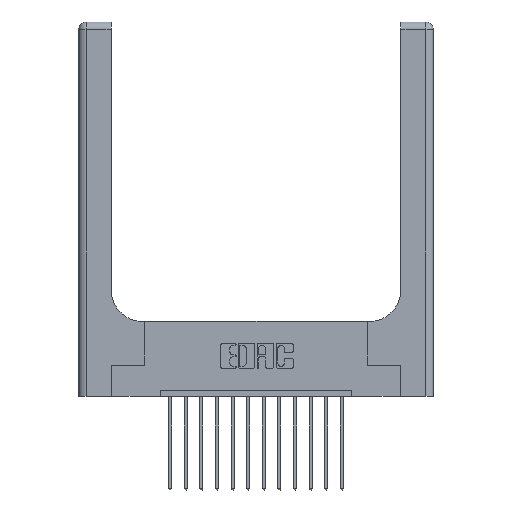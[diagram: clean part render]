
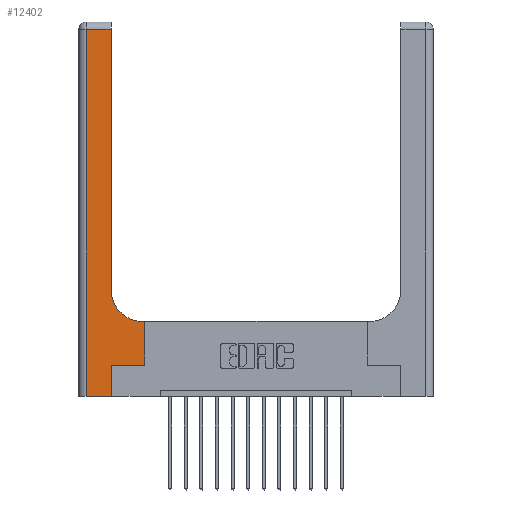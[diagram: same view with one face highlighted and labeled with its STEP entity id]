
A CAD part, top view. The second image highlights one B-rep face of the part: STEP entity #12402.
In plain terms, the highlighted planar face has unit normal (0, 0, 1).
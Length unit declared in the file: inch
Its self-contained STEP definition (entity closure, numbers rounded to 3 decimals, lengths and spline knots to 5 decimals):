
#96 = CARTESIAN_POINT ( 'NONE',  ( 0., 3., 0.37 ) ) ;
#171 = VERTEX_POINT ( 'NONE', #6019 ) ;
#181 = DIRECTION ( 'NONE',  ( 1., 0., 0. ) ) ;
#257 = EDGE_CURVE ( 'NONE', #2579, #5908, #6985, .T. ) ;
#1175 = LINE ( 'NONE', #15353, #2236 ) ;
#1240 = CARTESIAN_POINT ( 'NONE',  ( 0.528, 0.25, 0.37 ) ) ;
#1268 = CARTESIAN_POINT ( 'NONE',  ( 0.26, 2.94, 0.37 ) ) ;
#1392 = PLANE ( 'NONE',  #9883 ) ;
#1414 = ORIENTED_EDGE ( 'NONE', *, *, #13776, .T. ) ;
#1678 = LINE ( 'NONE', #4248, #4530 ) ;
#2134 = DIRECTION ( 'NONE',  ( 0., -1., 0. ) ) ;
#2166 = EDGE_CURVE ( 'NONE', #8527, #7662, #1175, .T. ) ;
#2236 = VECTOR ( 'NONE', #16609, 39.37008 ) ;
#2522 = VERTEX_POINT ( 'NONE', #14238 ) ;
#2579 = VERTEX_POINT ( 'NONE', #14970 ) ;
#2643 = CARTESIAN_POINT ( 'NONE',  ( 0.528, 0.25, 0.37 ) ) ;
#2962 = EDGE_CURVE ( 'NONE', #5908, #13254, #7901, .T. ) ;
#3064 = FACE_OUTER_BOUND ( 'NONE', #5101, .T. ) ;
#3127 = VECTOR ( 'NONE', #8066, 39.37008 ) ;
#3618 = VECTOR ( 'NONE', #3876, 39.37008 ) ;
#3773 = LINE ( 'NONE', #7328, #7438 ) ;
#3876 = DIRECTION ( 'NONE',  ( 0., 1., 0. ) ) ;
#4155 = EDGE_CURVE ( 'NONE', #171, #8527, #4359, .T. ) ;
#4224 = ORIENTED_EDGE ( 'NONE', *, *, #257, .T. ) ;
#4248 = CARTESIAN_POINT ( 'NONE',  ( 0., 0., 0.37 ) ) ;
#4333 = EDGE_CURVE ( 'NONE', #16553, #2522, #3773, .T. ) ;
#4359 = CIRCLE ( 'NONE', #16296, 0.25 ) ;
#4530 = VECTOR ( 'NONE', #14507, 39.37008 ) ;
#4594 = DIRECTION ( 'NONE',  ( 0., 1., 0. ) ) ;
#5101 = EDGE_LOOP ( 'NONE', ( #5566, #12782, #16397, #5996, #15455, #4224, #14226, #1414, #9257 ) ) ;
#5499 = DIRECTION ( 'NONE',  ( -1., 0., 0. ) ) ;
#5566 = ORIENTED_EDGE ( 'NONE', *, *, #2166, .T. ) ;
#5616 = CARTESIAN_POINT ( 'NONE',  ( 0.265, 0., 0.37 ) ) ;
#5675 = CARTESIAN_POINT ( 'NONE',  ( 0.06, 2.94, 0.37 ) ) ;
#5908 = VERTEX_POINT ( 'NONE', #2643 ) ;
#5996 = ORIENTED_EDGE ( 'NONE', *, *, #10366, .T. ) ;
#6019 = CARTESIAN_POINT ( 'NONE',  ( 0.51, 0.6, 0.37 ) ) ;
#6820 = LINE ( 'NONE', #13614, #12020 ) ;
#6902 = CARTESIAN_POINT ( 'NONE',  ( 0.528, 0.6, 0.37 ) ) ;
#6924 = VERTEX_POINT ( 'NONE', #5616 ) ;
#6932 = DIRECTION ( 'NONE',  ( -1., 0., 0. ) ) ;
#6985 = LINE ( 'NONE', #15513, #3127 ) ;
#7328 = CARTESIAN_POINT ( 'NONE',  ( 0.06, 3., 0.37 ) ) ;
#7438 = VECTOR ( 'NONE', #2134, 39.37008 ) ;
#7662 = VERTEX_POINT ( 'NONE', #1268 ) ;
#7901 = LINE ( 'NONE', #1240, #3618 ) ;
#7954 = DIRECTION ( 'NONE',  ( 0., 0., -1. ) ) ;
#8066 = DIRECTION ( 'NONE',  ( 1., 0., 0. ) ) ;
#8527 = VERTEX_POINT ( 'NONE', #9975 ) ;
#9257 = ORIENTED_EDGE ( 'NONE', *, *, #4155, .T. ) ;
#9510 = VECTOR ( 'NONE', #6932, 39.37008 ) ;
#9733 = CARTESIAN_POINT ( 'NONE',  ( 0., 2.94, 0.37 ) ) ;
#9795 = EDGE_CURVE ( 'NONE', #6924, #2579, #6820, .T. ) ;
#9883 = AXIS2_PLACEMENT_3D ( 'NONE', #96, #7954, #5499 ) ;
#9944 = EDGE_CURVE ( 'NONE', #7662, #16553, #12790, .T. ) ;
#9975 = CARTESIAN_POINT ( 'NONE',  ( 0.26, 0.85, 0.37 ) ) ;
#10212 = DIRECTION ( 'NONE',  ( -1., 0., 0. ) ) ;
#10366 = EDGE_CURVE ( 'NONE', #2522, #6924, #1678, .T. ) ;
#11564 = DIRECTION ( 'NONE',  ( 0., 0., -1. ) ) ;
#12007 = VECTOR ( 'NONE', #10212, 39.37008 ) ;
#12020 = VECTOR ( 'NONE', #4594, 39.37008 ) ;
#12402 = ADVANCED_FACE ( 'NONE', ( #3064 ), #1392, .F. ) ;
#12782 = ORIENTED_EDGE ( 'NONE', *, *, #9944, .T. ) ;
#12790 = LINE ( 'NONE', #9733, #12007 ) ;
#12943 = CARTESIAN_POINT ( 'NONE',  ( 0.51, 0.85, 0.37 ) ) ;
#13254 = VERTEX_POINT ( 'NONE', #6902 ) ;
#13614 = CARTESIAN_POINT ( 'NONE',  ( 0.265, 0., 0.37 ) ) ;
#13776 = EDGE_CURVE ( 'NONE', #13254, #171, #13861, .T. ) ;
#13861 = LINE ( 'NONE', #14551, #9510 ) ;
#14226 = ORIENTED_EDGE ( 'NONE', *, *, #2962, .T. ) ;
#14238 = CARTESIAN_POINT ( 'NONE',  ( 0.06, 0., 0.37 ) ) ;
#14507 = DIRECTION ( 'NONE',  ( 1., 0., 0. ) ) ;
#14551 = CARTESIAN_POINT ( 'NONE',  ( 0.26, 0.6, 0.37 ) ) ;
#14970 = CARTESIAN_POINT ( 'NONE',  ( 0.265, 0.25, 0.37 ) ) ;
#15353 = CARTESIAN_POINT ( 'NONE',  ( 0.26, 3., 0.37 ) ) ;
#15455 = ORIENTED_EDGE ( 'NONE', *, *, #9795, .T. ) ;
#15513 = CARTESIAN_POINT ( 'NONE',  ( 0.265, 0.25, 0.37 ) ) ;
#16296 = AXIS2_PLACEMENT_3D ( 'NONE', #12943, #11564, #181 ) ;
#16397 = ORIENTED_EDGE ( 'NONE', *, *, #4333, .T. ) ;
#16553 = VERTEX_POINT ( 'NONE', #5675 ) ;
#16609 = DIRECTION ( 'NONE',  ( 0., 1., 0. ) ) ;
